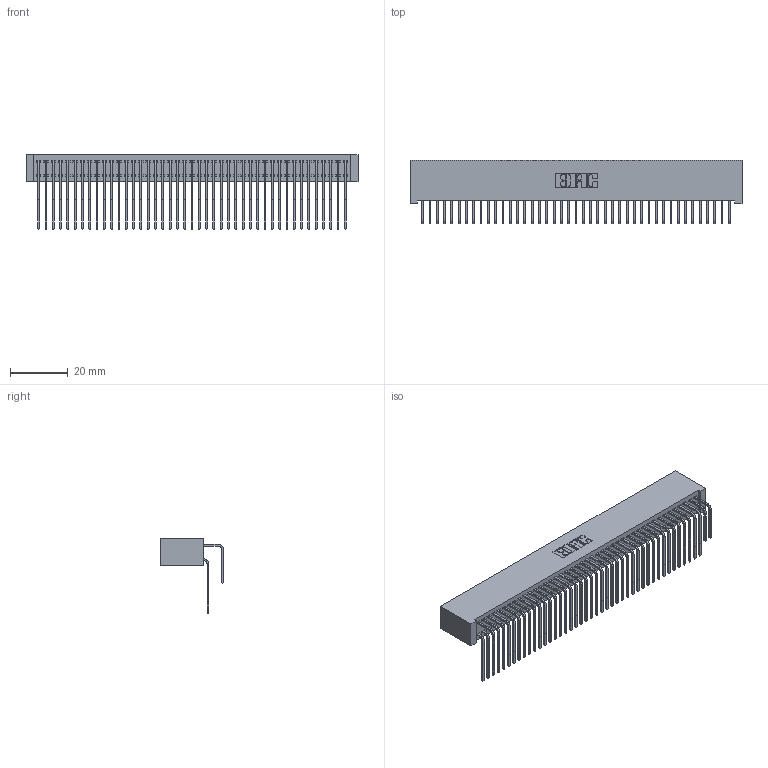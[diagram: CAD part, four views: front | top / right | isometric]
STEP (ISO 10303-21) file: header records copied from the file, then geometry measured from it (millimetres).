
FILE_DESCRIPTION (( 'STEP AP203' ), '1' );
FILE_NAME ('392-086-558-201.STEP', '2019-10-09T16:26:25', ( '' ), ( '' ), 'SwSTEP 2.0', 'SolidWorks 2016', '' );
FILE_SCHEMA (( 'CONFIG_CONTROL_DESIGN' ));
Length unit declared in the file: inch
Products named in the file (4): 342 Part_Lugless; 345-292-001_558 559 Tail - 1; 345-292-001_558 Tail - 2; 392-086-558-201
Assembly tree (87 placements, depth 2):
  392-086-558-201
    342 Part_Lugless
    345-292-001_558 559 Tail - 1  x43
    345-292-001_558 Tail - 2  x43
Bounding box: 115.47 x 21.91 x 25.78 mm (x, y, z)
Volume: 11315.2 mm3; surface area: 21133.4 mm2
Topology: 87 solids, 87 shells, 4746 faces, 14121 edges, 9298 vertices
Faces by surface type: plane 3330, cylinder 1416
Entity records: 28909 total; most frequent: CARTESIAN_POINT 4837, ORIENTED_EDGE 4722, DIRECTION 4105, EDGE_CURVE 2361, VECTOR 2201, LINE 2201, VERTEX_POINT 1570, AXIS2_PLACEMENT_3D 952
